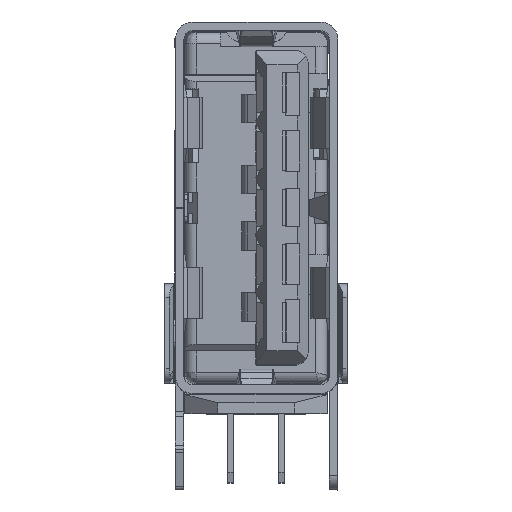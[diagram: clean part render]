
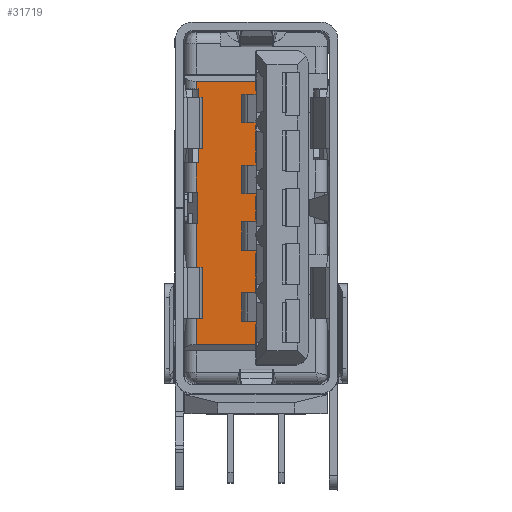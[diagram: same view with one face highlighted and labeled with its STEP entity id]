
A CAD part, top view. The second image highlights one B-rep face of the part: STEP entity #31719.
In plain terms, the highlighted planar face has unit normal (0, 0, 1).
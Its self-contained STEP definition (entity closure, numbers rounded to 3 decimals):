
#108 = LINE ( 'NONE', #85558, #38554 ) ;
#1069 = EDGE_CURVE ( 'NONE', #12779, #92569, #14717, .T. ) ;
#1120 = ORIENTED_EDGE ( 'NONE', *, *, #54974, .T. ) ;
#3073 = EDGE_CURVE ( 'NONE', #86414, #6605, #83039, .T. ) ;
#4063 = VECTOR ( 'NONE', #91585, 1000. ) ;
#6260 = LINE ( 'NONE', #34904, #76484 ) ;
#6605 = VERTEX_POINT ( 'NONE', #85693 ) ;
#6918 = LINE ( 'NONE', #49636, #57379 ) ;
#7663 = CARTESIAN_POINT ( 'NONE',  ( -2.04, -0.17, -10.48 ) ) ;
#8187 = ORIENTED_EDGE ( 'NONE', *, *, #54151, .T. ) ;
#8973 = CARTESIAN_POINT ( 'NONE',  ( -2.11, -0.55, -10.48 ) ) ;
#12779 = VERTEX_POINT ( 'NONE', #32331 ) ;
#14072 = ORIENTED_EDGE ( 'NONE', *, *, #80224, .T. ) ;
#14386 = ORIENTED_EDGE ( 'NONE', *, *, #20524, .T. ) ;
#14584 = DIRECTION ( 'NONE',  ( 1., 0., 0. ) ) ;
#14709 = CARTESIAN_POINT ( 'NONE',  ( 0., -4.57, -10.48 ) ) ;
#14717 = LINE ( 'NONE', #7663, #49050 ) ;
#14972 = ORIENTED_EDGE ( 'NONE', *, *, #1069, .T. ) ;
#15504 = VERTEX_POINT ( 'NONE', #15993 ) ;
#15993 = CARTESIAN_POINT ( 'NONE',  ( -2.11, 0.55, -10.48 ) ) ;
#16315 = DIRECTION ( 'NONE',  ( 0., 0., 1. ) ) ;
#20524 = EDGE_CURVE ( 'NONE', #45462, #15504, #55377, .T. ) ;
#22304 = CARTESIAN_POINT ( 'NONE',  ( -1.055, -0.55, -10.48 ) ) ;
#22644 = CARTESIAN_POINT ( 'NONE',  ( -2.11, 4.2, -10.48 ) ) ;
#24709 = CARTESIAN_POINT ( 'NONE',  ( 0., -4.81, -10.48 ) ) ;
#25293 = DIRECTION ( 'NONE',  ( 0., -1., 0. ) ) ;
#26896 = EDGE_CURVE ( 'NONE', #43105, #82018, #62995, .T. ) ;
#28329 = VECTOR ( 'NONE', #56374, 1000. ) ;
#29357 = VECTOR ( 'NONE', #71590, 1000. ) ;
#29833 = VERTEX_POINT ( 'NONE', #40417 ) ;
#29887 = ORIENTED_EDGE ( 'NONE', *, *, #32896, .T. ) ;
#31719 = ADVANCED_FACE ( 'NONE', ( #44942 ), #51071, .T. ) ;
#32331 = CARTESIAN_POINT ( 'NONE',  ( -2.04, 4.2, -10.48 ) ) ;
#32896 = EDGE_CURVE ( 'NONE', #61183, #43105, #108, .T. ) ;
#33843 = LINE ( 'NONE', #92554, #28329 ) ;
#34904 = CARTESIAN_POINT ( 'NONE',  ( -2.275, 1.6, -10.48 ) ) ;
#35401 = EDGE_CURVE ( 'NONE', #29833, #86414, #50473, .T. ) ;
#35552 = DIRECTION ( 'NONE',  ( 0., 1., 0. ) ) ;
#36265 = ORIENTED_EDGE ( 'NONE', *, *, #35401, .T. ) ;
#36348 = EDGE_CURVE ( 'NONE', #42138, #61183, #43836, .T. ) ;
#38554 = VECTOR ( 'NONE', #49850, 1000. ) ;
#40417 = CARTESIAN_POINT ( 'NONE',  ( -2.05, -0.55, -10.48 ) ) ;
#42138 = VERTEX_POINT ( 'NONE', #14709 ) ;
#42588 = CARTESIAN_POINT ( 'NONE',  ( -2.05, 0., -10.48 ) ) ;
#43105 = VERTEX_POINT ( 'NONE', #51992 ) ;
#43329 = DIRECTION ( 'NONE',  ( -1., 0., 0. ) ) ;
#43836 = LINE ( 'NONE', #78621, #29357 ) ;
#44942 = FACE_OUTER_BOUND ( 'NONE', #48201, .T. ) ;
#45400 = CARTESIAN_POINT ( 'NONE',  ( 0.042, -4.996, -10.48 ) ) ;
#45462 = VERTEX_POINT ( 'NONE', #88104 ) ;
#45908 = AXIS2_PLACEMENT_3D ( 'NONE', #45400, #16315, #81132 ) ;
#46044 = LINE ( 'NONE', #68126, #4063 ) ;
#46284 = ORIENTED_EDGE ( 'NONE', *, *, #26896, .T. ) ;
#46940 = VECTOR ( 'NONE', #86424, 1000. ) ;
#47860 = CARTESIAN_POINT ( 'NONE',  ( -2.11, 1.075, -10.48 ) ) ;
#48201 = EDGE_LOOP ( 'NONE', ( #56690, #53085, #29887, #46284, #14072, #14972, #1120, #14386, #55671, #70982, #36265, #80305, #8187 ) ) ;
#49050 = VECTOR ( 'NONE', #64992, 1000. ) ;
#49636 = CARTESIAN_POINT ( 'NONE',  ( -1.055, 0.55, -10.48 ) ) ;
#49850 = DIRECTION ( 'NONE',  ( -1., 0., 0. ) ) ;
#50473 = LINE ( 'NONE', #22304, #86684 ) ;
#51071 = PLANE ( 'NONE',  #45908 ) ;
#51992 = CARTESIAN_POINT ( 'NONE',  ( -2.11, 4.47, -10.48 ) ) ;
#53085 = ORIENTED_EDGE ( 'NONE', *, *, #36348, .T. ) ;
#54151 = EDGE_CURVE ( 'NONE', #6605, #60587, #56855, .T. ) ;
#54974 = EDGE_CURVE ( 'NONE', #92569, #45462, #6260, .T. ) ;
#55377 = LINE ( 'NONE', #47860, #74936 ) ;
#55671 = ORIENTED_EDGE ( 'NONE', *, *, #69864, .T. ) ;
#56374 = DIRECTION ( 'NONE',  ( 0., 1., 0. ) ) ;
#56690 = ORIENTED_EDGE ( 'NONE', *, *, #83488, .T. ) ;
#56855 = LINE ( 'NONE', #92561, #79374 ) ;
#57157 = LINE ( 'NONE', #42588, #63433 ) ;
#57379 = VECTOR ( 'NONE', #65151, 1000. ) ;
#60587 = VERTEX_POINT ( 'NONE', #24709 ) ;
#61183 = VERTEX_POINT ( 'NONE', #77477 ) ;
#61634 = VERTEX_POINT ( 'NONE', #79231 ) ;
#62995 = LINE ( 'NONE', #71893, #46940 ) ;
#63433 = VECTOR ( 'NONE', #35552, 1000. ) ;
#64992 = DIRECTION ( 'NONE',  ( 0., -1., 0. ) ) ;
#65151 = DIRECTION ( 'NONE',  ( 1., 0., 0. ) ) ;
#68126 = CARTESIAN_POINT ( 'NONE',  ( -2.275, 4.2, -10.48 ) ) ;
#69864 = EDGE_CURVE ( 'NONE', #15504, #61634, #6918, .T. ) ;
#69920 = EDGE_CURVE ( 'NONE', #29833, #61634, #57157, .T. ) ;
#70982 = ORIENTED_EDGE ( 'NONE', *, *, #69920, .F. ) ;
#71590 = DIRECTION ( 'NONE',  ( 0., 1., 0. ) ) ;
#71893 = CARTESIAN_POINT ( 'NONE',  ( -2.11, -0.17, -10.48 ) ) ;
#74611 = CARTESIAN_POINT ( 'NONE',  ( -2.11, -2.76, -10.48 ) ) ;
#74936 = VECTOR ( 'NONE', #91087, 1000. ) ;
#76484 = VECTOR ( 'NONE', #43329, 1000. ) ;
#77477 = CARTESIAN_POINT ( 'NONE',  ( 0., 4.47, -10.48 ) ) ;
#78621 = CARTESIAN_POINT ( 'NONE',  ( 0., -0.17, -10.48 ) ) ;
#79132 = DIRECTION ( 'NONE',  ( -1., 0., 0. ) ) ;
#79231 = CARTESIAN_POINT ( 'NONE',  ( -2.05, 0.55, -10.48 ) ) ;
#79374 = VECTOR ( 'NONE', #14584, 1000. ) ;
#80224 = EDGE_CURVE ( 'NONE', #82018, #12779, #46044, .T. ) ;
#80305 = ORIENTED_EDGE ( 'NONE', *, *, #3073, .T. ) ;
#81132 = DIRECTION ( 'NONE',  ( 0., 1., 0. ) ) ;
#81562 = CARTESIAN_POINT ( 'NONE',  ( -2.04, 1.6, -10.48 ) ) ;
#82018 = VERTEX_POINT ( 'NONE', #22644 ) ;
#83039 = LINE ( 'NONE', #74611, #84154 ) ;
#83488 = EDGE_CURVE ( 'NONE', #60587, #42138, #33843, .T. ) ;
#84154 = VECTOR ( 'NONE', #25293, 1000. ) ;
#85558 = CARTESIAN_POINT ( 'NONE',  ( -1.055, 4.47, -10.48 ) ) ;
#85693 = CARTESIAN_POINT ( 'NONE',  ( -2.11, -4.81, -10.48 ) ) ;
#86414 = VERTEX_POINT ( 'NONE', #8973 ) ;
#86424 = DIRECTION ( 'NONE',  ( 0., -1., 0. ) ) ;
#86684 = VECTOR ( 'NONE', #79132, 1000. ) ;
#88104 = CARTESIAN_POINT ( 'NONE',  ( -2.11, 1.6, -10.48 ) ) ;
#91087 = DIRECTION ( 'NONE',  ( 0., -1., 0. ) ) ;
#91585 = DIRECTION ( 'NONE',  ( 1., 0., 0. ) ) ;
#92554 = CARTESIAN_POINT ( 'NONE',  ( 0., -0.17, -10.48 ) ) ;
#92561 = CARTESIAN_POINT ( 'NONE',  ( -1.055, -4.81, -10.48 ) ) ;
#92569 = VERTEX_POINT ( 'NONE', #81562 ) ;
